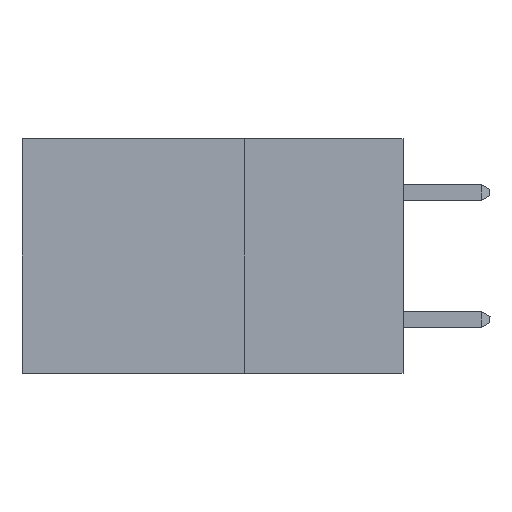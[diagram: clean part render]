
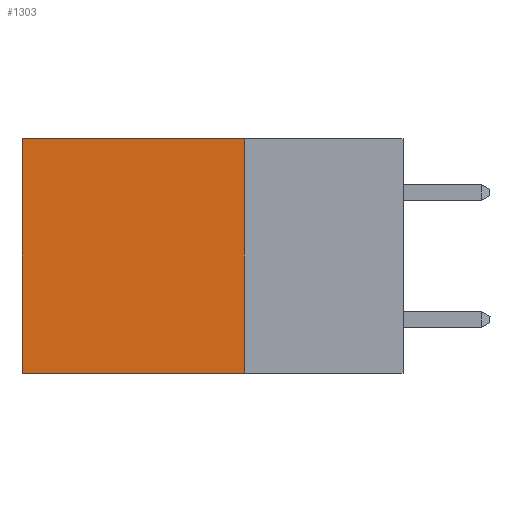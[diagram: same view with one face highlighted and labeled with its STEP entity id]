
A CAD part, left-side view. The second image highlights one B-rep face of the part: STEP entity #1303.
In plain terms, the highlighted planar face has unit normal (-1, 0, 0).
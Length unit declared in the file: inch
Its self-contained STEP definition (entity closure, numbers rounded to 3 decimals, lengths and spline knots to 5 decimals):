
#89 = DIRECTION ( 'NONE',  ( 0., 1., 0. ) ) ;
#340 = CARTESIAN_POINT ( 'NONE',  ( 0.2875, 0.25, 0. ) ) ;
#786 = DIRECTION ( 'NONE',  ( 0., 1., 0. ) ) ;
#1303 = ADVANCED_FACE ( 'NONE', ( #15010 ), #2493, .F. ) ;
#1526 = CARTESIAN_POINT ( 'NONE',  ( 0.2875, 0.25, 0. ) ) ;
#1692 = VERTEX_POINT ( 'NONE', #4143 ) ;
#2368 = VECTOR ( 'NONE', #3355, 39.37008 ) ;
#2493 = PLANE ( 'NONE',  #8460 ) ;
#3029 = CARTESIAN_POINT ( 'NONE',  ( 0.2875, 0.6, 0. ) ) ;
#3355 = DIRECTION ( 'NONE',  ( 0., 0., -1. ) ) ;
#3897 = VECTOR ( 'NONE', #13818, 39.37008 ) ;
#4143 = CARTESIAN_POINT ( 'NONE',  ( 0.2875, 0.6, -0.37 ) ) ;
#4550 = EDGE_CURVE ( 'NONE', #14925, #12430, #6630, .T. ) ;
#4750 = ORIENTED_EDGE ( 'NONE', *, *, #4550, .T. ) ;
#6368 = CARTESIAN_POINT ( 'NONE',  ( 0.2875, 0.25, 0. ) ) ;
#6630 = LINE ( 'NONE', #14094, #9677 ) ;
#7622 = ORIENTED_EDGE ( 'NONE', *, *, #11008, .F. ) ;
#8460 = AXIS2_PLACEMENT_3D ( 'NONE', #1526, #14935, #8757 ) ;
#8501 = CARTESIAN_POINT ( 'NONE',  ( 0.2875, 0.25, -0.37 ) ) ;
#8757 = DIRECTION ( 'NONE',  ( 0., 0., -1. ) ) ;
#9317 = CARTESIAN_POINT ( 'NONE',  ( 0.2875, 0.25, -0.37 ) ) ;
#9462 = CARTESIAN_POINT ( 'NONE',  ( 0.2875, 0.6, 0. ) ) ;
#9509 = VECTOR ( 'NONE', #89, 39.37008 ) ;
#9677 = VECTOR ( 'NONE', #786, 39.37008 ) ;
#10527 = EDGE_CURVE ( 'NONE', #15039, #1692, #13710, .T. ) ;
#10742 = ORIENTED_EDGE ( 'NONE', *, *, #12224, .T. ) ;
#11008 = EDGE_CURVE ( 'NONE', #14925, #15039, #13515, .T. ) ;
#11700 = EDGE_LOOP ( 'NONE', ( #10742, #15642, #7622, #4750 ) ) ;
#11874 = LINE ( 'NONE', #9462, #2368 ) ;
#12224 = EDGE_CURVE ( 'NONE', #12430, #1692, #11874, .T. ) ;
#12430 = VERTEX_POINT ( 'NONE', #3029 ) ;
#13515 = LINE ( 'NONE', #6368, #3897 ) ;
#13710 = LINE ( 'NONE', #8501, #9509 ) ;
#13818 = DIRECTION ( 'NONE',  ( 0., 0., -1. ) ) ;
#14094 = CARTESIAN_POINT ( 'NONE',  ( 0.2875, 0.25, 0. ) ) ;
#14925 = VERTEX_POINT ( 'NONE', #340 ) ;
#14935 = DIRECTION ( 'NONE',  ( 1., 0., 0. ) ) ;
#15010 = FACE_OUTER_BOUND ( 'NONE', #11700, .T. ) ;
#15039 = VERTEX_POINT ( 'NONE', #9317 ) ;
#15642 = ORIENTED_EDGE ( 'NONE', *, *, #10527, .F. ) ;
